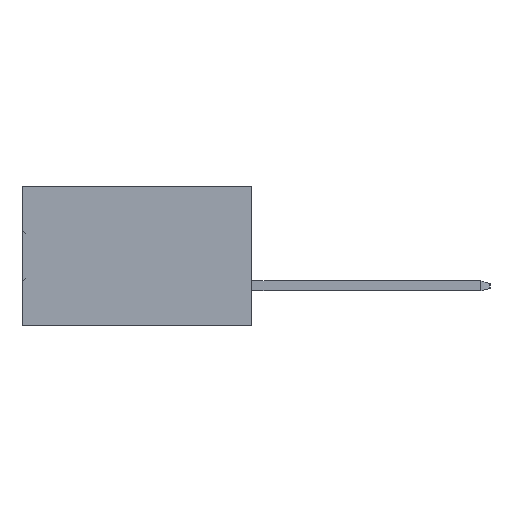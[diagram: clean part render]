
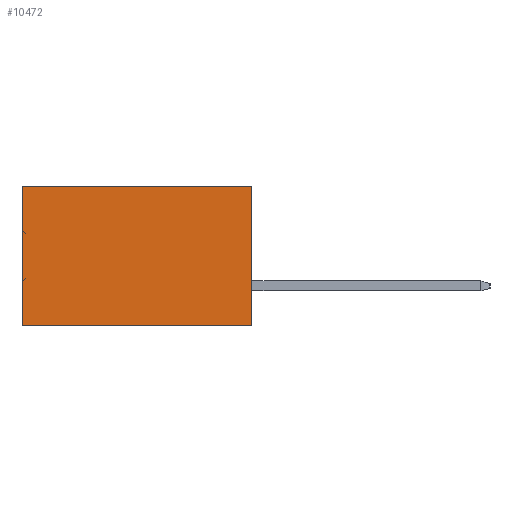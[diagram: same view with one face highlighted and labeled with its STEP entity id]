
A CAD part, left-side view. The second image highlights one B-rep face of the part: STEP entity #10472.
In plain terms, the highlighted planar face has unit normal (-1, 0, 0).
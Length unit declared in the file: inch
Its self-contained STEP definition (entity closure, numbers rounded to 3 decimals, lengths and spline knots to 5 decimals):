
#304 = VERTEX_POINT ( 'NONE', #19694 ) ;
#766 = FACE_OUTER_BOUND ( 'NONE', #23094, .T. ) ;
#1044 = CARTESIAN_POINT ( 'NONE',  ( 0.3205, 0.72, 0. ) ) ;
#1129 = EDGE_CURVE ( 'NONE', #14341, #17583, #6470, .T. ) ;
#1481 = DIRECTION ( 'NONE',  ( 0., 1., 0. ) ) ;
#3245 = CARTESIAN_POINT ( 'NONE',  ( 0.3205, 0., -0.437 ) ) ;
#5733 = DIRECTION ( 'NONE',  ( 0., 1., 0. ) ) ;
#6470 = LINE ( 'NONE', #16127, #27836 ) ;
#7215 = CARTESIAN_POINT ( 'NONE',  ( 0.3205, 0., -0.437 ) ) ;
#7755 = LINE ( 'NONE', #17238, #29137 ) ;
#7904 = EDGE_CURVE ( 'NONE', #304, #20312, #7755, .T. ) ;
#9112 = CARTESIAN_POINT ( 'NONE',  ( 0.3205, 0., 0. ) ) ;
#9854 = EDGE_CURVE ( 'NONE', #14341, #304, #12037, .T. ) ;
#10259 = PLANE ( 'NONE',  #16467 ) ;
#10472 = ADVANCED_FACE ( 'NONE', ( #766 ), #10259, .F. ) ;
#11460 = VECTOR ( 'NONE', #21321, 39.37008 ) ;
#12037 = LINE ( 'NONE', #7215, #11460 ) ;
#12755 = DIRECTION ( 'NONE',  ( 1., 0., 0. ) ) ;
#14341 = VERTEX_POINT ( 'NONE', #9112 ) ;
#15122 = ORIENTED_EDGE ( 'NONE', *, *, #9854, .F. ) ;
#15130 = VECTOR ( 'NONE', #16897, 39.37008 ) ;
#15494 = EDGE_CURVE ( 'NONE', #17583, #20312, #21678, .T. ) ;
#16127 = CARTESIAN_POINT ( 'NONE',  ( 0.3205, 0., 0. ) ) ;
#16467 = AXIS2_PLACEMENT_3D ( 'NONE', #3245, #12755, #22158 ) ;
#16897 = DIRECTION ( 'NONE',  ( 0., 0., -1. ) ) ;
#17238 = CARTESIAN_POINT ( 'NONE',  ( 0.3205, 0., -0.437 ) ) ;
#17344 = CARTESIAN_POINT ( 'NONE',  ( 0.3205, 0.72, -0.437 ) ) ;
#17583 = VERTEX_POINT ( 'NONE', #1044 ) ;
#19694 = CARTESIAN_POINT ( 'NONE',  ( 0.3205, 0., -0.437 ) ) ;
#20312 = VERTEX_POINT ( 'NONE', #25234 ) ;
#21321 = DIRECTION ( 'NONE',  ( 0., 0., -1. ) ) ;
#21678 = LINE ( 'NONE', #17344, #15130 ) ;
#22158 = DIRECTION ( 'NONE',  ( 0., 0., -1. ) ) ;
#23094 = EDGE_LOOP ( 'NONE', ( #28441, #27854, #15122, #28305 ) ) ;
#25234 = CARTESIAN_POINT ( 'NONE',  ( 0.3205, 0.72, -0.437 ) ) ;
#27836 = VECTOR ( 'NONE', #1481, 39.37008 ) ;
#27854 = ORIENTED_EDGE ( 'NONE', *, *, #7904, .F. ) ;
#28305 = ORIENTED_EDGE ( 'NONE', *, *, #1129, .T. ) ;
#28441 = ORIENTED_EDGE ( 'NONE', *, *, #15494, .T. ) ;
#29137 = VECTOR ( 'NONE', #5733, 39.37008 ) ;
